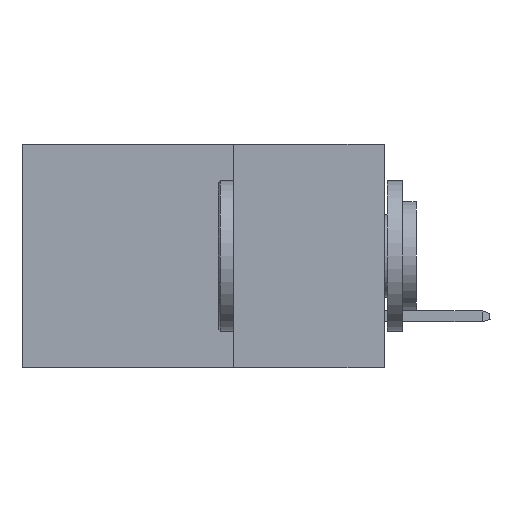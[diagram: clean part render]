
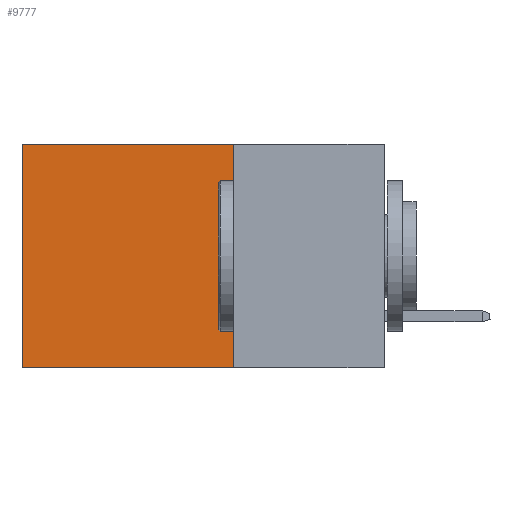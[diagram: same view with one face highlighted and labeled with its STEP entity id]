
A CAD part, left-side view. The second image highlights one B-rep face of the part: STEP entity #9777.
In plain terms, the highlighted planar face has unit normal (-1, 0, 0).
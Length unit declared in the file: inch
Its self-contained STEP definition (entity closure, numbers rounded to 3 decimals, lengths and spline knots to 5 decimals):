
#360 = PLANE ( 'NONE',  #476 ) ;
#476 = AXIS2_PLACEMENT_3D ( 'NONE', #23978, #10153, #24066 ) ;
#2824 = DIRECTION ( 'NONE',  ( 0., 1., 0. ) ) ;
#5207 = ORIENTED_EDGE ( 'NONE', *, *, #25313, .F. ) ;
#5532 = CARTESIAN_POINT ( 'NONE',  ( 0.298, 0.6, 0. ) ) ;
#5736 = LINE ( 'NONE', #6626, #10444 ) ;
#5785 = LINE ( 'NONE', #18167, #25720 ) ;
#6626 = CARTESIAN_POINT ( 'NONE',  ( 0.298, 0.25, 0. ) ) ;
#6923 = VERTEX_POINT ( 'NONE', #24476 ) ;
#7488 = LINE ( 'NONE', #23792, #17459 ) ;
#7599 = EDGE_LOOP ( 'NONE', ( #21191, #15853, #5207, #14508 ) ) ;
#8398 = VECTOR ( 'NONE', #25004, 39.37008 ) ;
#8401 = VERTEX_POINT ( 'NONE', #5532 ) ;
#8661 = EDGE_CURVE ( 'NONE', #8401, #19255, #25520, .T. ) ;
#9777 = ADVANCED_FACE ( 'NONE', ( #19542 ), #360, .F. ) ;
#10153 = DIRECTION ( 'NONE',  ( 1., 0., 0. ) ) ;
#10430 = EDGE_CURVE ( 'NONE', #11548, #19255, #5785, .T. ) ;
#10444 = VECTOR ( 'NONE', #2824, 39.37008 ) ;
#11150 = EDGE_CURVE ( 'NONE', #6923, #8401, #5736, .T. ) ;
#11548 = VERTEX_POINT ( 'NONE', #14503 ) ;
#12217 = DIRECTION ( 'NONE',  ( 0., 0., -1. ) ) ;
#13962 = CARTESIAN_POINT ( 'NONE',  ( 0.298, 0.6, -0.37 ) ) ;
#14503 = CARTESIAN_POINT ( 'NONE',  ( 0.298, 0.25, -0.37 ) ) ;
#14508 = ORIENTED_EDGE ( 'NONE', *, *, #11150, .T. ) ;
#15853 = ORIENTED_EDGE ( 'NONE', *, *, #10430, .F. ) ;
#17459 = VECTOR ( 'NONE', #12217, 39.37008 ) ;
#18167 = CARTESIAN_POINT ( 'NONE',  ( 0.298, 0.25, -0.37 ) ) ;
#19255 = VERTEX_POINT ( 'NONE', #13962 ) ;
#19542 = FACE_OUTER_BOUND ( 'NONE', #7599, .T. ) ;
#21191 = ORIENTED_EDGE ( 'NONE', *, *, #8661, .T. ) ;
#22736 = CARTESIAN_POINT ( 'NONE',  ( 0.298, 0.6, 0. ) ) ;
#23792 = CARTESIAN_POINT ( 'NONE',  ( 0.298, 0.25, 0. ) ) ;
#23922 = DIRECTION ( 'NONE',  ( 0., 1., 0. ) ) ;
#23978 = CARTESIAN_POINT ( 'NONE',  ( 0.298, 0.25, 0. ) ) ;
#24066 = DIRECTION ( 'NONE',  ( 0., 0., -1. ) ) ;
#24476 = CARTESIAN_POINT ( 'NONE',  ( 0.298, 0.25, 0. ) ) ;
#25004 = DIRECTION ( 'NONE',  ( 0., 0., -1. ) ) ;
#25313 = EDGE_CURVE ( 'NONE', #6923, #11548, #7488, .T. ) ;
#25520 = LINE ( 'NONE', #22736, #8398 ) ;
#25720 = VECTOR ( 'NONE', #23922, 39.37008 ) ;
